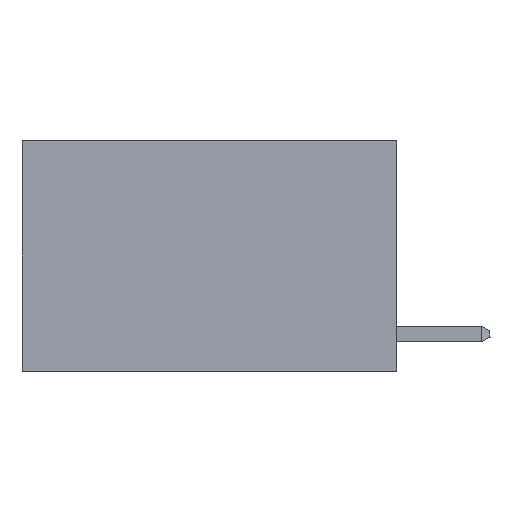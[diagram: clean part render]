
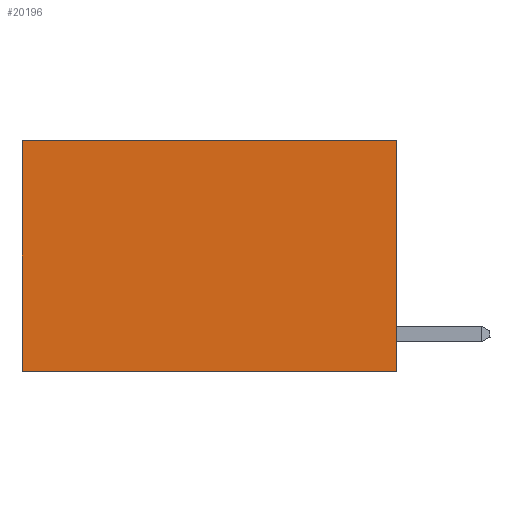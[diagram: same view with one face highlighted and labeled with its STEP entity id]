
A CAD part, left-side view. The second image highlights one B-rep face of the part: STEP entity #20196.
In plain terms, the highlighted planar face has unit normal (-1, 0, 0).
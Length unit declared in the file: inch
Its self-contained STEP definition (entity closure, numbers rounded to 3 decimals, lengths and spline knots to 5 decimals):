
#90 = LINE ( 'NONE', #17709, #10582 ) ;
#392 = DIRECTION ( 'NONE',  ( 0., 1., 0. ) ) ;
#609 = LINE ( 'NONE', #6992, #17052 ) ;
#2268 = EDGE_LOOP ( 'NONE', ( #13102, #23935, #20904, #5151 ) ) ;
#2361 = VERTEX_POINT ( 'NONE', #4948 ) ;
#2625 = EDGE_CURVE ( 'NONE', #20084, #14190, #90, .T. ) ;
#4653 = CARTESIAN_POINT ( 'NONE',  ( 0.2625, 0., 0. ) ) ;
#4948 = CARTESIAN_POINT ( 'NONE',  ( 0.2625, 0.6, -0.37 ) ) ;
#5151 = ORIENTED_EDGE ( 'NONE', *, *, #18978, .T. ) ;
#5986 = LINE ( 'NONE', #26052, #23085 ) ;
#6992 = CARTESIAN_POINT ( 'NONE',  ( 0.2625, 0., 0. ) ) ;
#7580 = CARTESIAN_POINT ( 'NONE',  ( 0.2625, 0., -0.37 ) ) ;
#8256 = DIRECTION ( 'NONE',  ( 0., 0., -1. ) ) ;
#9017 = DIRECTION ( 'NONE',  ( 1., 0., 0. ) ) ;
#10582 = VECTOR ( 'NONE', #17026, 39.37008 ) ;
#11521 = AXIS2_PLACEMENT_3D ( 'NONE', #4653, #9017, #23962 ) ;
#12041 = VERTEX_POINT ( 'NONE', #19973 ) ;
#12446 = LINE ( 'NONE', #16694, #23157 ) ;
#13102 = ORIENTED_EDGE ( 'NONE', *, *, #18122, .T. ) ;
#14190 = VERTEX_POINT ( 'NONE', #7580 ) ;
#16694 = CARTESIAN_POINT ( 'NONE',  ( 0.2625, 0.6, 0. ) ) ;
#17026 = DIRECTION ( 'NONE',  ( 0., 0., -1. ) ) ;
#17052 = VECTOR ( 'NONE', #24205, 39.37008 ) ;
#17511 = PLANE ( 'NONE',  #11521 ) ;
#17709 = CARTESIAN_POINT ( 'NONE',  ( 0.2625, 0., 0. ) ) ;
#18122 = EDGE_CURVE ( 'NONE', #12041, #2361, #12446, .T. ) ;
#18978 = EDGE_CURVE ( 'NONE', #20084, #12041, #609, .T. ) ;
#19687 = FACE_OUTER_BOUND ( 'NONE', #2268, .T. ) ;
#19973 = CARTESIAN_POINT ( 'NONE',  ( 0.2625, 0.6, 0. ) ) ;
#20084 = VERTEX_POINT ( 'NONE', #25654 ) ;
#20196 = ADVANCED_FACE ( 'NONE', ( #19687 ), #17511, .F. ) ;
#20904 = ORIENTED_EDGE ( 'NONE', *, *, #2625, .F. ) ;
#22503 = EDGE_CURVE ( 'NONE', #14190, #2361, #5986, .T. ) ;
#23085 = VECTOR ( 'NONE', #392, 39.37008 ) ;
#23157 = VECTOR ( 'NONE', #8256, 39.37008 ) ;
#23935 = ORIENTED_EDGE ( 'NONE', *, *, #22503, .F. ) ;
#23962 = DIRECTION ( 'NONE',  ( 0., 0., -1. ) ) ;
#24205 = DIRECTION ( 'NONE',  ( 0., 1., 0. ) ) ;
#25654 = CARTESIAN_POINT ( 'NONE',  ( 0.2625, 0., 0. ) ) ;
#26052 = CARTESIAN_POINT ( 'NONE',  ( 0.2625, 0., -0.37 ) ) ;
